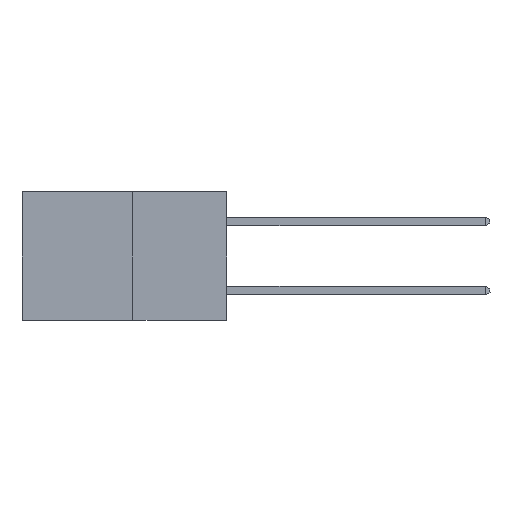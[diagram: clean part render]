
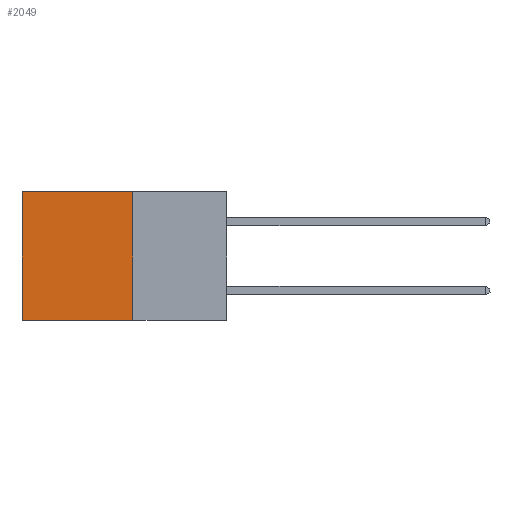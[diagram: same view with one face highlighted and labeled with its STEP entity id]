
A CAD part, left-side view. The second image highlights one B-rep face of the part: STEP entity #2049.
In plain terms, the highlighted planar face has unit normal (-1, 0, 0).
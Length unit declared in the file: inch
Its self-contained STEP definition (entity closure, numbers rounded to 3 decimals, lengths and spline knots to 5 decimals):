
#529 = CARTESIAN_POINT ( 'NONE',  ( 0.277, 0.27, -0.37 ) ) ;
#1078 = CARTESIAN_POINT ( 'NONE',  ( 0.277, 0.27, -0.37 ) ) ;
#2049 = ADVANCED_FACE ( 'NONE', ( #31087 ), #7317, .F. ) ;
#3623 = CARTESIAN_POINT ( 'NONE',  ( 0.277, 0.59, -0.37 ) ) ;
#5352 = AXIS2_PLACEMENT_3D ( 'NONE', #529, #13234, #10658 ) ;
#6781 = VECTOR ( 'NONE', #24396, 39.37008 ) ;
#7317 = PLANE ( 'NONE',  #5352 ) ;
#8388 = ORIENTED_EDGE ( 'NONE', *, *, #29790, .T. ) ;
#9467 = VERTEX_POINT ( 'NONE', #3623 ) ;
#9839 = CARTESIAN_POINT ( 'NONE',  ( 0.277, 0.59, -0.37 ) ) ;
#10504 = VECTOR ( 'NONE', #31606, 39.37008 ) ;
#10658 = DIRECTION ( 'NONE',  ( 0., 0., -1. ) ) ;
#10816 = LINE ( 'NONE', #1078, #28827 ) ;
#12134 = CARTESIAN_POINT ( 'NONE',  ( 0.277, 0.27, -0.37 ) ) ;
#13234 = DIRECTION ( 'NONE',  ( 1., 0., 0. ) ) ;
#14473 = ORIENTED_EDGE ( 'NONE', *, *, #26016, .F. ) ;
#15728 = VECTOR ( 'NONE', #24795, 39.37008 ) ;
#16509 = LINE ( 'NONE', #9839, #15728 ) ;
#16792 = VERTEX_POINT ( 'NONE', #17203 ) ;
#17203 = CARTESIAN_POINT ( 'NONE',  ( 0.277, 0.27, -0.37 ) ) ;
#18707 = EDGE_CURVE ( 'NONE', #16792, #9467, #10816, .T. ) ;
#20126 = LINE ( 'NONE', #21941, #6781 ) ;
#20982 = EDGE_LOOP ( 'NONE', ( #22211, #28115, #14473, #8388 ) ) ;
#21184 = DIRECTION ( 'NONE',  ( 0., 1., 0. ) ) ;
#21941 = CARTESIAN_POINT ( 'NONE',  ( 0.277, 0.27, 0. ) ) ;
#22211 = ORIENTED_EDGE ( 'NONE', *, *, #24718, .T. ) ;
#24396 = DIRECTION ( 'NONE',  ( 0., 1., 0. ) ) ;
#24718 = EDGE_CURVE ( 'NONE', #26703, #9467, #16509, .T. ) ;
#24795 = DIRECTION ( 'NONE',  ( 0., 0., -1. ) ) ;
#26016 = EDGE_CURVE ( 'NONE', #28745, #16792, #30044, .T. ) ;
#26269 = CARTESIAN_POINT ( 'NONE',  ( 0.277, 0.59, 0. ) ) ;
#26483 = CARTESIAN_POINT ( 'NONE',  ( 0.277, 0.27, 0. ) ) ;
#26703 = VERTEX_POINT ( 'NONE', #26269 ) ;
#28115 = ORIENTED_EDGE ( 'NONE', *, *, #18707, .F. ) ;
#28745 = VERTEX_POINT ( 'NONE', #26483 ) ;
#28827 = VECTOR ( 'NONE', #21184, 39.37008 ) ;
#29790 = EDGE_CURVE ( 'NONE', #28745, #26703, #20126, .T. ) ;
#30044 = LINE ( 'NONE', #12134, #10504 ) ;
#31087 = FACE_OUTER_BOUND ( 'NONE', #20982, .T. ) ;
#31606 = DIRECTION ( 'NONE',  ( 0., 0., -1. ) ) ;
